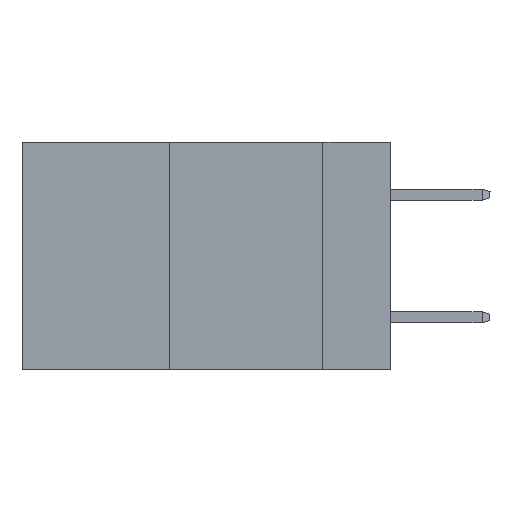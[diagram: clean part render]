
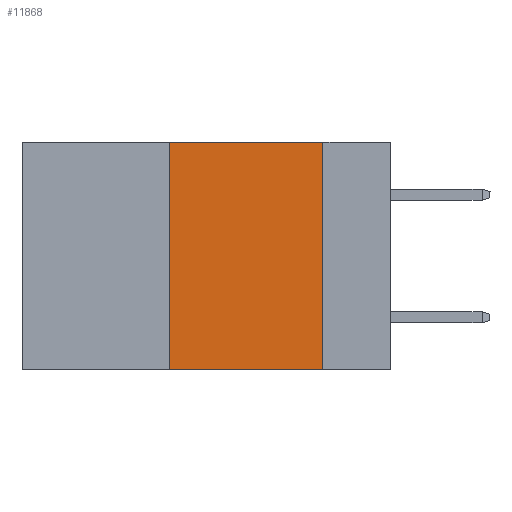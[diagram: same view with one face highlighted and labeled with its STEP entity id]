
A CAD part, left-side view. The second image highlights one B-rep face of the part: STEP entity #11868.
In plain terms, the highlighted planar face has unit normal (-1, 0, 0).
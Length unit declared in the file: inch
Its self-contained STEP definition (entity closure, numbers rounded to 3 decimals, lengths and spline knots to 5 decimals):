
#388 = VECTOR ( 'NONE', #21120, 39.37008 ) ;
#1012 = CARTESIAN_POINT ( 'NONE',  ( 0., 0.6, -0.37 ) ) ;
#1791 = VECTOR ( 'NONE', #21556, 39.37008 ) ;
#2711 = LINE ( 'NONE', #1012, #21953 ) ;
#3051 = ORIENTED_EDGE ( 'NONE', *, *, #17011, .F. ) ;
#3589 = EDGE_CURVE ( 'NONE', #9111, #21650, #2711, .T. ) ;
#3912 = DIRECTION ( 'NONE',  ( 1., 0., 0. ) ) ;
#4318 = EDGE_CURVE ( 'NONE', #9111, #17770, #22791, .T. ) ;
#4748 = AXIS2_PLACEMENT_3D ( 'NONE', #20428, #3912, #22021 ) ;
#4872 = DIRECTION ( 'NONE',  ( 0., -1., 0. ) ) ;
#6400 = EDGE_LOOP ( 'NONE', ( #14972, #3051, #16084, #23653 ) ) ;
#6749 = CARTESIAN_POINT ( 'NONE',  ( 0., 0.36, -0.37 ) ) ;
#6825 = CARTESIAN_POINT ( 'NONE',  ( 0., 0.11, 0. ) ) ;
#9111 = VERTEX_POINT ( 'NONE', #6749 ) ;
#11468 = DIRECTION ( 'NONE',  ( 0., 0., 1. ) ) ;
#11699 = CARTESIAN_POINT ( 'NONE',  ( 0., 0.36, 0. ) ) ;
#11868 = ADVANCED_FACE ( 'NONE', ( #14662 ), #13091, .F. ) ;
#13091 = PLANE ( 'NONE',  #4748 ) ;
#13860 = VERTEX_POINT ( 'NONE', #17056 ) ;
#14662 = FACE_OUTER_BOUND ( 'NONE', #6400, .T. ) ;
#14972 = ORIENTED_EDGE ( 'NONE', *, *, #23627, .F. ) ;
#15291 = CARTESIAN_POINT ( 'NONE',  ( 0., 0.11, -0.37 ) ) ;
#15769 = LINE ( 'NONE', #6825, #1791 ) ;
#16084 = ORIENTED_EDGE ( 'NONE', *, *, #4318, .F. ) ;
#16848 = VECTOR ( 'NONE', #11468, 39.37008 ) ;
#17011 = EDGE_CURVE ( 'NONE', #17770, #13860, #23174, .T. ) ;
#17056 = CARTESIAN_POINT ( 'NONE',  ( 0., 0.11, 0. ) ) ;
#17770 = VERTEX_POINT ( 'NONE', #21376 ) ;
#19547 = CARTESIAN_POINT ( 'NONE',  ( 0., 0.6, 0. ) ) ;
#20428 = CARTESIAN_POINT ( 'NONE',  ( 0., 0.6, 0. ) ) ;
#21120 = DIRECTION ( 'NONE',  ( 0., -1., 0. ) ) ;
#21376 = CARTESIAN_POINT ( 'NONE',  ( 0., 0.36, 0. ) ) ;
#21556 = DIRECTION ( 'NONE',  ( 0., 0., -1. ) ) ;
#21650 = VERTEX_POINT ( 'NONE', #15291 ) ;
#21953 = VECTOR ( 'NONE', #4872, 39.37008 ) ;
#22021 = DIRECTION ( 'NONE',  ( 0., 0., -1. ) ) ;
#22791 = LINE ( 'NONE', #11699, #16848 ) ;
#23174 = LINE ( 'NONE', #19547, #388 ) ;
#23627 = EDGE_CURVE ( 'NONE', #13860, #21650, #15769, .T. ) ;
#23653 = ORIENTED_EDGE ( 'NONE', *, *, #3589, .T. ) ;
